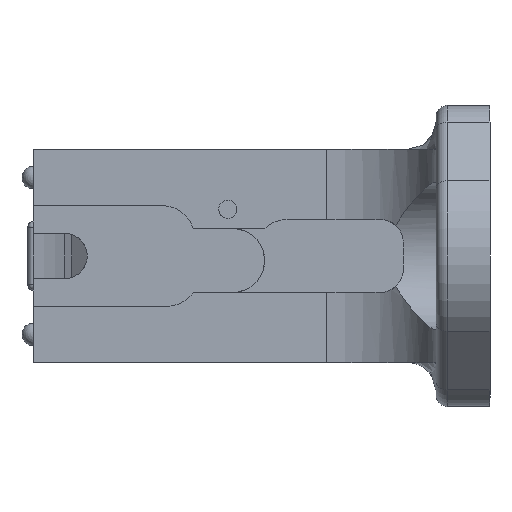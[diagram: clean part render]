
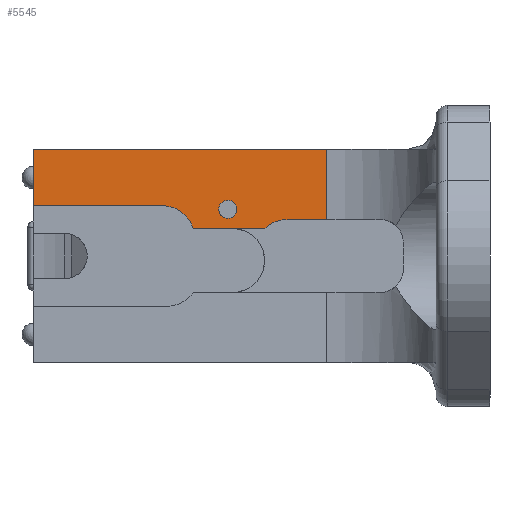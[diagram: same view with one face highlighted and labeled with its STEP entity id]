
A CAD part, left-side view. The second image highlights one B-rep face of the part: STEP entity #5545.
In plain terms, the highlighted planar face has unit normal (-1, 0, 0).
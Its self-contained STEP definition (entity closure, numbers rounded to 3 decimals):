
#129 = CARTESIAN_POINT ( 'NONE',  ( -90.918, -145.831, 10.897 ) ) ;
#206 = EDGE_CURVE ( 'NONE', #3260, #10471, #10323, .T. ) ;
#574 = DIRECTION ( 'NONE',  ( 0., 0., -1. ) ) ;
#662 = DIRECTION ( 'NONE',  ( 0., 0., 1. ) ) ;
#1060 = CARTESIAN_POINT ( 'NONE',  ( -90.918, -287.36, 11.096 ) ) ;
#1476 = VECTOR ( 'NONE', #7675, 1000. ) ;
#1649 = VERTEX_POINT ( 'NONE', #6261 ) ;
#1673 = VERTEX_POINT ( 'NONE', #7140 ) ;
#1771 = CARTESIAN_POINT ( 'NONE',  ( -90.918, -145.831, 9.323 ) ) ;
#1966 = DIRECTION ( 'NONE',  ( 1., 0., 0. ) ) ;
#2081 = EDGE_CURVE ( 'NONE', #6242, #1673, #5978, .T. ) ;
#2148 = CARTESIAN_POINT ( 'NONE',  ( -90.918, -145.831, -9.74 ) ) ;
#2375 = EDGE_CURVE ( 'NONE', #5214, #8146, #3844, .T. ) ;
#2488 = CARTESIAN_POINT ( 'NONE',  ( -90.918, -281.315, 9.323 ) ) ;
#2695 = ORIENTED_EDGE ( 'NONE', *, *, #206, .T. ) ;
#2706 = DIRECTION ( 'NONE',  ( 1., 0., 0. ) ) ;
#2765 = CARTESIAN_POINT ( 'NONE',  ( -90.918, -253.472, -855.789 ) ) ;
#3052 = CARTESIAN_POINT ( 'NONE',  ( -90.918, -94.3, 23.114 ) ) ;
#3156 = FACE_OUTER_BOUND ( 'NONE', #8516, .T. ) ;
#3243 = AXIS2_PLACEMENT_3D ( 'NONE', #2148, #3794, #9749 ) ;
#3260 = VERTEX_POINT ( 'NONE', #9577 ) ;
#3424 = FACE_BOUND ( 'NONE', #4969, .T. ) ;
#3469 = DIRECTION ( 'NONE',  ( 0., -1., 0. ) ) ;
#3716 = LINE ( 'NONE', #1771, #1476 ) ;
#3732 = DIRECTION ( 'NONE',  ( 0., 1., 0. ) ) ;
#3794 = DIRECTION ( 'NONE',  ( -1., 0., 0. ) ) ;
#3844 = CIRCLE ( 'NONE', #3998, 5.556 ) ;
#3977 = VECTOR ( 'NONE', #8943, 1000. ) ;
#3998 = AXIS2_PLACEMENT_3D ( 'NONE', #7033, #1966, #7887 ) ;
#4253 = VECTOR ( 'NONE', #3469, 1000. ) ;
#4382 = ORIENTED_EDGE ( 'NONE', *, *, #5989, .T. ) ;
#4470 = DIRECTION ( 'NONE',  ( 0., 0., -1. ) ) ;
#4701 = ORIENTED_EDGE ( 'NONE', *, *, #7343, .F. ) ;
#4840 = ORIENTED_EDGE ( 'NONE', *, *, #2375, .T. ) ;
#4969 = EDGE_LOOP ( 'NONE', ( #4382 ) ) ;
#5203 = VERTEX_POINT ( 'NONE', #6259 ) ;
#5211 = ORIENTED_EDGE ( 'NONE', *, *, #8311, .T. ) ;
#5214 = VERTEX_POINT ( 'NONE', #8784 ) ;
#5272 = CIRCLE ( 'NONE', #9238, 1.587 ) ;
#5545 = ADVANCED_FACE ( 'NONE', ( #3424, #3156 ), #8906, .T. ) ;
#5604 = VECTOR ( 'NONE', #4470, 1000. ) ;
#5634 = DIRECTION ( 'NONE',  ( 1., 0., 0. ) ) ;
#5704 = CARTESIAN_POINT ( 'NONE',  ( -90.918, -253.472, 13.31 ) ) ;
#5714 = CARTESIAN_POINT ( 'NONE',  ( -90.918, -304.581, -13.919 ) ) ;
#5978 = LINE ( 'NONE', #129, #4253 ) ;
#5989 = EDGE_CURVE ( 'NONE', #9750, #9750, #5272, .T. ) ;
#6081 = CIRCLE ( 'NONE', #10283, 5.556 ) ;
#6180 = CARTESIAN_POINT ( 'NONE',  ( -90.918, -297.662, 10.897 ) ) ;
#6223 = LINE ( 'NONE', #3052, #3977 ) ;
#6242 = VERTEX_POINT ( 'NONE', #6180 ) ;
#6259 = CARTESIAN_POINT ( 'NONE',  ( -90.918, -293.786, 9.323 ) ) ;
#6261 = CARTESIAN_POINT ( 'NONE',  ( -90.918, -304.581, 23.114 ) ) ;
#6633 = VECTOR ( 'NONE', #662, 1000. ) ;
#6926 = ORIENTED_EDGE ( 'NONE', *, *, #9731, .T. ) ;
#7033 = CARTESIAN_POINT ( 'NONE',  ( -90.918, -275.985, 7.754 ) ) ;
#7091 = LINE ( 'NONE', #9619, #9060 ) ;
#7140 = CARTESIAN_POINT ( 'NONE',  ( -90.918, -304.581, 10.897 ) ) ;
#7343 = EDGE_CURVE ( 'NONE', #5214, #10471, #7091, .T. ) ;
#7675 = DIRECTION ( 'NONE',  ( 0., 1., 0. ) ) ;
#7777 = CARTESIAN_POINT ( 'NONE',  ( -90.918, -297.662, 5.341 ) ) ;
#7887 = DIRECTION ( 'NONE',  ( 0., -1., 0. ) ) ;
#8146 = VERTEX_POINT ( 'NONE', #2488 ) ;
#8311 = EDGE_CURVE ( 'NONE', #1673, #1649, #8858, .T. ) ;
#8516 = EDGE_LOOP ( 'NONE', ( #5211, #6926, #2695, #4701, #4840, #10853, #10371, #9195 ) ) ;
#8609 = DIRECTION ( 'NONE',  ( 0., -1., 0. ) ) ;
#8784 = CARTESIAN_POINT ( 'NONE',  ( -90.918, -275.985, 13.31 ) ) ;
#8858 = LINE ( 'NONE', #5714, #6633 ) ;
#8906 = PLANE ( 'NONE',  #3243 ) ;
#8943 = DIRECTION ( 'NONE',  ( 0., 1., 0. ) ) ;
#8956 = EDGE_CURVE ( 'NONE', #5203, #8146, #3716, .T. ) ;
#9060 = VECTOR ( 'NONE', #3732, 1000. ) ;
#9195 = ORIENTED_EDGE ( 'NONE', *, *, #2081, .T. ) ;
#9238 = AXIS2_PLACEMENT_3D ( 'NONE', #10651, #5634, #574 ) ;
#9577 = CARTESIAN_POINT ( 'NONE',  ( -90.918, -253.472, 23.114 ) ) ;
#9619 = CARTESIAN_POINT ( 'NONE',  ( -90.918, -145.831, 13.31 ) ) ;
#9731 = EDGE_CURVE ( 'NONE', #1649, #3260, #6223, .T. ) ;
#9749 = DIRECTION ( 'NONE',  ( 0., -1., 0. ) ) ;
#9750 = VERTEX_POINT ( 'NONE', #1060 ) ;
#10283 = AXIS2_PLACEMENT_3D ( 'NONE', #7777, #2706, #8609 ) ;
#10323 = LINE ( 'NONE', #2765, #5604 ) ;
#10371 = ORIENTED_EDGE ( 'NONE', *, *, #10911, .T. ) ;
#10471 = VERTEX_POINT ( 'NONE', #5704 ) ;
#10651 = CARTESIAN_POINT ( 'NONE',  ( -90.918, -287.36, 12.683 ) ) ;
#10853 = ORIENTED_EDGE ( 'NONE', *, *, #8956, .F. ) ;
#10911 = EDGE_CURVE ( 'NONE', #5203, #6242, #6081, .T. ) ;
